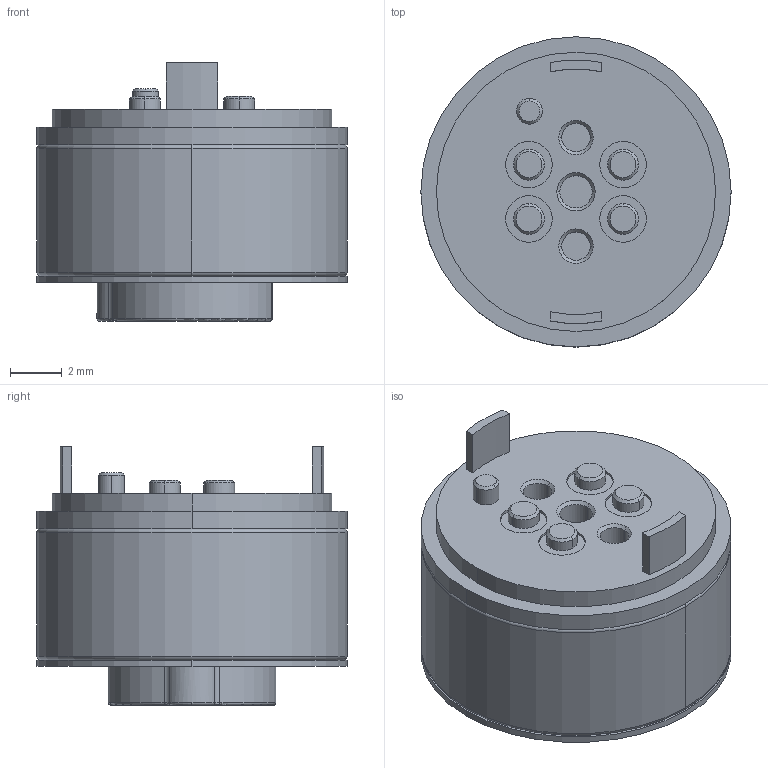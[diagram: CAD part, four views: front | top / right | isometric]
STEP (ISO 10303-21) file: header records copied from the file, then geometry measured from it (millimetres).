
FILE_DESCRIPTION (( 'STEP AP203' ), '1' );
FILE_NAME ('686-A04222A01E1.STEP', '2023-02-03T17:12:58', ( 'Magnum' ), ( '' ), 'SwSTEP 2.0', 'SolidWorks 2020', '' );
FILE_SCHEMA (( 'CONFIG_CONTROL_DESIGN' ));
Length unit declared in the file: millimetre
Products named in the file (1): 686-A04222A01E1
Bounding box: 12 x 12 x 10 mm (x, y, z)
Volume: 784.9 mm3; surface area: 638.3 mm2
Topology: 5 solids, 7 shells, 332 faces, 840 edges, 542 vertices
Faces by surface type: plane 147, cylinder 95, bspline 36, cone 34, torus 16, sphere 4
Entity records: 11998 total; most frequent: CARTESIAN_POINT 4085, ORIENTED_EDGE 1660, DIRECTION 1564, EDGE_CURVE 830, AXIS2_PLACEMENT_3D 564, VERTEX_POINT 542, VECTOR 436, LINE 436
